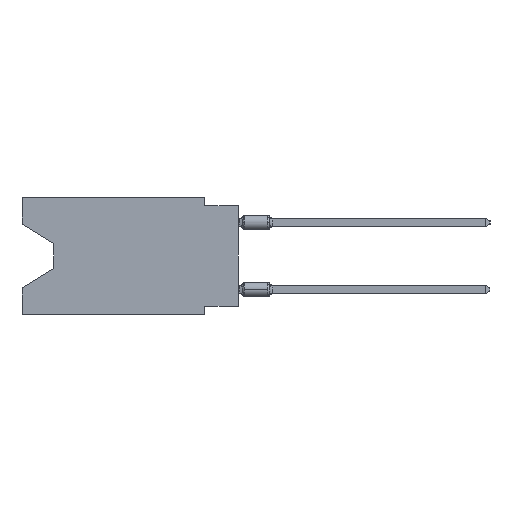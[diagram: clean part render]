
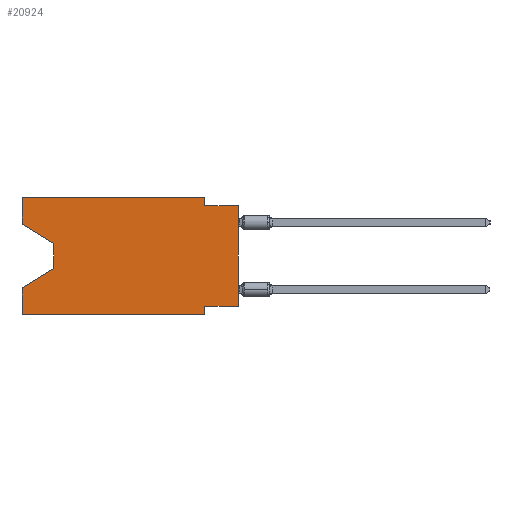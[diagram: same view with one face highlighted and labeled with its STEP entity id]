
A CAD part, left-side view. The second image highlights one B-rep face of the part: STEP entity #20924.
In plain terms, the highlighted planar face has unit normal (-1, 0, 0).
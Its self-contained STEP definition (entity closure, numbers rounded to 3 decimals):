
#624 = ORIENTED_EDGE ( 'NONE', *, *, #4150, .F. ) ;
#792 = VECTOR ( 'NONE', #5497, 1000. ) ;
#823 = VERTEX_POINT ( 'NONE', #42728 ) ;
#1464 = EDGE_CURVE ( 'NONE', #21945, #26694, #43736, .T. ) ;
#2713 = ORIENTED_EDGE ( 'NONE', *, *, #22150, .F. ) ;
#3043 = CARTESIAN_POINT ( 'NONE',  ( 0., 16.383, 0. ) ) ;
#3203 = AXIS2_PLACEMENT_3D ( 'NONE', #4920, #8291, #18827 ) ;
#3543 = VECTOR ( 'NONE', #13787, 1000. ) ;
#3657 = CARTESIAN_POINT ( 'NONE',  ( 0., 16.383, -2.038 ) ) ;
#4111 = LINE ( 'NONE', #38491, #5695 ) ;
#4150 = EDGE_CURVE ( 'NONE', #11236, #44017, #35349, .T. ) ;
#4501 = EDGE_LOOP ( 'NONE', ( #20100, #41938, #43618, #23768, #33515, #26957, #16766, #11267, #624, #29023, #2713, #15326 ) ) ;
#4920 = CARTESIAN_POINT ( 'NONE',  ( 0., 16.383, 0. ) ) ;
#5158 = FACE_OUTER_BOUND ( 'NONE', #4501, .T. ) ;
#5497 = DIRECTION ( 'NONE',  ( 0., 1., 0. ) ) ;
#5695 = VECTOR ( 'NONE', #11964, 1000. ) ;
#6273 = LINE ( 'NONE', #31181, #36893 ) ;
#6335 = VECTOR ( 'NONE', #22830, 1000. ) ;
#6461 = DIRECTION ( 'NONE',  ( 0., 0., 1. ) ) ;
#8266 = VECTOR ( 'NONE', #20572, 1000. ) ;
#8291 = DIRECTION ( 'NONE',  ( 1., 0., 0. ) ) ;
#8485 = CARTESIAN_POINT ( 'NONE',  ( 0., 13.97, -5.385 ) ) ;
#9080 = LINE ( 'NONE', #19175, #792 ) ;
#9590 = LINE ( 'NONE', #37197, #17054 ) ;
#11236 = VERTEX_POINT ( 'NONE', #17699 ) ;
#11267 = ORIENTED_EDGE ( 'NONE', *, *, #34707, .T. ) ;
#11665 = PLANE ( 'NONE',  #3203 ) ;
#11964 = DIRECTION ( 'NONE',  ( 0., 0., 1. ) ) ;
#12572 = CARTESIAN_POINT ( 'NONE',  ( 0., 2.54, -8.89 ) ) ;
#12677 = CARTESIAN_POINT ( 'NONE',  ( 0., 0., -0.635 ) ) ;
#13333 = CARTESIAN_POINT ( 'NONE',  ( 0., 2.54, 0. ) ) ;
#13757 = LINE ( 'NONE', #40954, #38322 ) ;
#13787 = DIRECTION ( 'NONE',  ( 0., 0., -1. ) ) ;
#13845 = LINE ( 'NONE', #43979, #8266 ) ;
#14329 = EDGE_CURVE ( 'NONE', #823, #23639, #4111, .T. ) ;
#15326 = ORIENTED_EDGE ( 'NONE', *, *, #1464, .F. ) ;
#16766 = ORIENTED_EDGE ( 'NONE', *, *, #23591, .F. ) ;
#16815 = CARTESIAN_POINT ( 'NONE',  ( 0., 16.383, -2.038 ) ) ;
#17054 = VECTOR ( 'NONE', #6461, 1000. ) ;
#17699 = CARTESIAN_POINT ( 'NONE',  ( 0., 2.54, -0.635 ) ) ;
#18827 = DIRECTION ( 'NONE',  ( 0., 0., -1. ) ) ;
#19175 = CARTESIAN_POINT ( 'NONE',  ( 0., 0., -8.255 ) ) ;
#19516 = VERTEX_POINT ( 'NONE', #27612 ) ;
#20100 = ORIENTED_EDGE ( 'NONE', *, *, #37262, .T. ) ;
#20398 = VERTEX_POINT ( 'NONE', #28389 ) ;
#20572 = DIRECTION ( 'NONE',  ( 0., -1., 0. ) ) ;
#20753 = DIRECTION ( 'NONE',  ( 0., -1., 0. ) ) ;
#20924 = ADVANCED_FACE ( 'NONE', ( #5158 ), #11665, .F. ) ;
#21945 = VERTEX_POINT ( 'NONE', #3657 ) ;
#22000 = EDGE_CURVE ( 'NONE', #34600, #23639, #13757, .T. ) ;
#22150 = EDGE_CURVE ( 'NONE', #26694, #35035, #6273, .T. ) ;
#22830 = DIRECTION ( 'NONE',  ( 0., 0., 1. ) ) ;
#23591 = EDGE_CURVE ( 'NONE', #30538, #43792, #9080, .T. ) ;
#23639 = VERTEX_POINT ( 'NONE', #30844 ) ;
#23768 = ORIENTED_EDGE ( 'NONE', *, *, #14329, .F. ) ;
#25129 = LINE ( 'NONE', #29135, #43548 ) ;
#25762 = CARTESIAN_POINT ( 'NONE',  ( 0., 0., -8.255 ) ) ;
#25806 = VECTOR ( 'NONE', #20753, 1000. ) ;
#26060 = DIRECTION ( 'NONE',  ( 0., 0., -1. ) ) ;
#26278 = DIRECTION ( 'NONE',  ( 0., -0.855, -0.519 ) ) ;
#26694 = VERTEX_POINT ( 'NONE', #41693 ) ;
#26957 = ORIENTED_EDGE ( 'NONE', *, *, #34189, .F. ) ;
#27612 = CARTESIAN_POINT ( 'NONE',  ( 0., 13.97, -3.505 ) ) ;
#28388 = CARTESIAN_POINT ( 'NONE',  ( 0., 0., -0.635 ) ) ;
#28389 = CARTESIAN_POINT ( 'NONE',  ( 0., 2.54, -8.89 ) ) ;
#29023 = ORIENTED_EDGE ( 'NONE', *, *, #36520, .F. ) ;
#29135 = CARTESIAN_POINT ( 'NONE',  ( 0., 13.97, -3.505 ) ) ;
#29369 = CARTESIAN_POINT ( 'NONE',  ( 0., 2.54, -8.255 ) ) ;
#30080 = LINE ( 'NONE', #16815, #34337 ) ;
#30538 = VERTEX_POINT ( 'NONE', #25762 ) ;
#30844 = CARTESIAN_POINT ( 'NONE',  ( 0., 16.383, -6.852 ) ) ;
#31181 = CARTESIAN_POINT ( 'NONE',  ( 0., 16.383, 0. ) ) ;
#31382 = VECTOR ( 'NONE', #26060, 1000. ) ;
#33314 = EDGE_CURVE ( 'NONE', #19516, #34600, #25129, .T. ) ;
#33515 = ORIENTED_EDGE ( 'NONE', *, *, #42628, .T. ) ;
#34189 = EDGE_CURVE ( 'NONE', #43792, #20398, #43373, .T. ) ;
#34337 = VECTOR ( 'NONE', #26278, 1000. ) ;
#34600 = VERTEX_POINT ( 'NONE', #8485 ) ;
#34707 = EDGE_CURVE ( 'NONE', #30538, #44017, #9590, .T. ) ;
#35035 = VERTEX_POINT ( 'NONE', #13333 ) ;
#35349 = LINE ( 'NONE', #28388, #25806 ) ;
#36520 = EDGE_CURVE ( 'NONE', #35035, #11236, #43701, .T. ) ;
#36893 = VECTOR ( 'NONE', #44034, 1000. ) ;
#37197 = CARTESIAN_POINT ( 'NONE',  ( 0., 0., 0. ) ) ;
#37262 = EDGE_CURVE ( 'NONE', #21945, #19516, #30080, .T. ) ;
#38322 = VECTOR ( 'NONE', #41177, 1000. ) ;
#38491 = CARTESIAN_POINT ( 'NONE',  ( 0., 16.383, 0. ) ) ;
#38826 = DIRECTION ( 'NONE',  ( 0., 0., -1. ) ) ;
#40532 = CARTESIAN_POINT ( 'NONE',  ( 0., 2.54, 0. ) ) ;
#40954 = CARTESIAN_POINT ( 'NONE',  ( 0., 13.97, -5.385 ) ) ;
#41177 = DIRECTION ( 'NONE',  ( 0., 0.855, -0.519 ) ) ;
#41693 = CARTESIAN_POINT ( 'NONE',  ( 0., 16.383, 0. ) ) ;
#41938 = ORIENTED_EDGE ( 'NONE', *, *, #33314, .T. ) ;
#42628 = EDGE_CURVE ( 'NONE', #823, #20398, #13845, .T. ) ;
#42728 = CARTESIAN_POINT ( 'NONE',  ( 0., 16.383, -8.89 ) ) ;
#43373 = LINE ( 'NONE', #12572, #31382 ) ;
#43548 = VECTOR ( 'NONE', #38826, 1000. ) ;
#43618 = ORIENTED_EDGE ( 'NONE', *, *, #22000, .T. ) ;
#43701 = LINE ( 'NONE', #40532, #3543 ) ;
#43736 = LINE ( 'NONE', #3043, #6335 ) ;
#43792 = VERTEX_POINT ( 'NONE', #29369 ) ;
#43979 = CARTESIAN_POINT ( 'NONE',  ( 0., 16.383, -8.89 ) ) ;
#44017 = VERTEX_POINT ( 'NONE', #12677 ) ;
#44034 = DIRECTION ( 'NONE',  ( 0., -1., 0. ) ) ;
